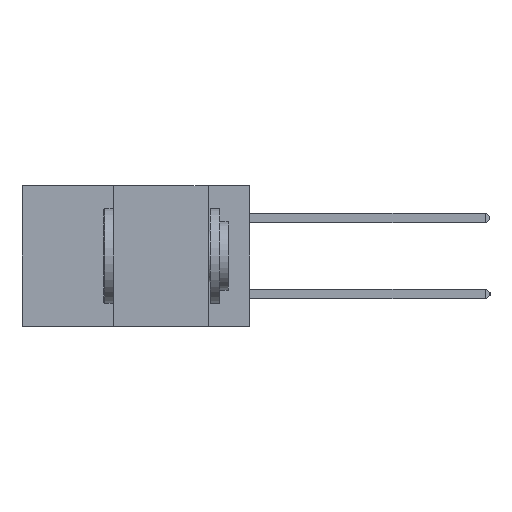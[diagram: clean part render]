
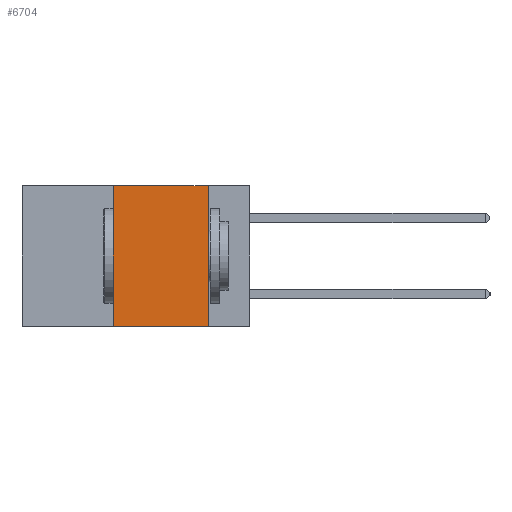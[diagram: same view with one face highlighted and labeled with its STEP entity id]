
A CAD part, left-side view. The second image highlights one B-rep face of the part: STEP entity #6704.
In plain terms, the highlighted planar face has unit normal (-1, 0, 0).
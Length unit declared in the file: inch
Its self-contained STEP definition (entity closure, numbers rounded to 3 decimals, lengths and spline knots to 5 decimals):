
#154 = EDGE_LOOP ( 'NONE', ( #10316, #4505, #4192, #755 ) ) ;
#251 = PLANE ( 'NONE',  #3868 ) ;
#755 = ORIENTED_EDGE ( 'NONE', *, *, #6961, .T. ) ;
#816 = VECTOR ( 'NONE', #4804, 39.37008 ) ;
#969 = VERTEX_POINT ( 'NONE', #11570 ) ;
#1423 = DIRECTION ( 'NONE',  ( 1., 0., 0. ) ) ;
#1760 = VECTOR ( 'NONE', #5874, 39.37008 ) ;
#2263 = CARTESIAN_POINT ( 'NONE',  ( 0., 0.11, -0.37 ) ) ;
#3552 = VERTEX_POINT ( 'NONE', #8189 ) ;
#3868 = AXIS2_PLACEMENT_3D ( 'NONE', #8336, #1423, #9394 ) ;
#3954 = LINE ( 'NONE', #11506, #816 ) ;
#4165 = VECTOR ( 'NONE', #9948, 39.37008 ) ;
#4192 = ORIENTED_EDGE ( 'NONE', *, *, #7736, .F. ) ;
#4505 = ORIENTED_EDGE ( 'NONE', *, *, #8625, .F. ) ;
#4612 = CARTESIAN_POINT ( 'NONE',  ( 0., 0.11, 0. ) ) ;
#4804 = DIRECTION ( 'NONE',  ( 0., -1., 0. ) ) ;
#4838 = LINE ( 'NONE', #10263, #1760 ) ;
#5874 = DIRECTION ( 'NONE',  ( 0., 0., 1. ) ) ;
#6704 = ADVANCED_FACE ( 'NONE', ( #11838 ), #251, .F. ) ;
#6961 = EDGE_CURVE ( 'NONE', #8262, #10495, #9929, .T. ) ;
#7736 = EDGE_CURVE ( 'NONE', #8262, #969, #4838, .T. ) ;
#8189 = CARTESIAN_POINT ( 'NONE',  ( 0., 0.11, 0. ) ) ;
#8262 = VERTEX_POINT ( 'NONE', #12113 ) ;
#8336 = CARTESIAN_POINT ( 'NONE',  ( 0., 0.6, 0. ) ) ;
#8459 = EDGE_CURVE ( 'NONE', #3552, #10495, #13672, .T. ) ;
#8625 = EDGE_CURVE ( 'NONE', #969, #3552, #3954, .T. ) ;
#9394 = DIRECTION ( 'NONE',  ( 0., 0., -1. ) ) ;
#9929 = LINE ( 'NONE', #12099, #4165 ) ;
#9948 = DIRECTION ( 'NONE',  ( 0., -1., 0. ) ) ;
#10263 = CARTESIAN_POINT ( 'NONE',  ( 0., 0.36, 0. ) ) ;
#10316 = ORIENTED_EDGE ( 'NONE', *, *, #8459, .F. ) ;
#10495 = VERTEX_POINT ( 'NONE', #2263 ) ;
#10942 = VECTOR ( 'NONE', #13362, 39.37008 ) ;
#11506 = CARTESIAN_POINT ( 'NONE',  ( 0., 0.6, 0. ) ) ;
#11570 = CARTESIAN_POINT ( 'NONE',  ( 0., 0.36, 0. ) ) ;
#11838 = FACE_OUTER_BOUND ( 'NONE', #154, .T. ) ;
#12099 = CARTESIAN_POINT ( 'NONE',  ( 0., 0.6, -0.37 ) ) ;
#12113 = CARTESIAN_POINT ( 'NONE',  ( 0., 0.36, -0.37 ) ) ;
#13362 = DIRECTION ( 'NONE',  ( 0., 0., -1. ) ) ;
#13672 = LINE ( 'NONE', #4612, #10942 ) ;
